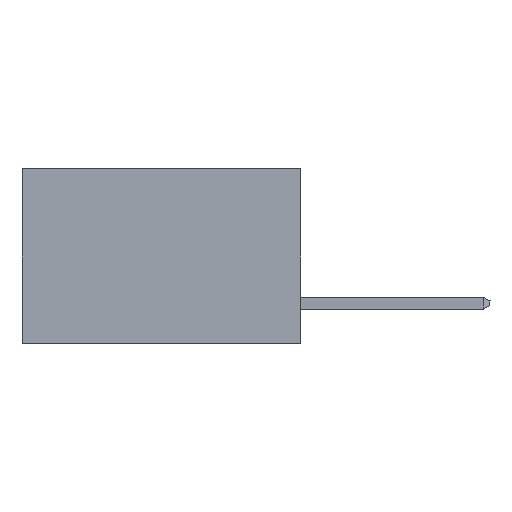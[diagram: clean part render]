
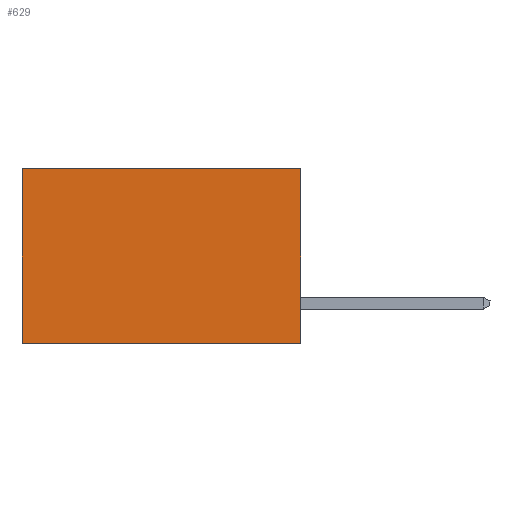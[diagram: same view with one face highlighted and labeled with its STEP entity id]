
A CAD part, left-side view. The second image highlights one B-rep face of the part: STEP entity #629.
In plain terms, the highlighted planar face has unit normal (-1, 0, 0).
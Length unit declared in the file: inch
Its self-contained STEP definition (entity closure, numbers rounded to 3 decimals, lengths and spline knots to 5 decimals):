
#10 = CARTESIAN_POINT ( 'NONE',  ( 0.277, 0., -0.37 ) ) ;
#412 = VECTOR ( 'NONE', #4377, 39.37008 ) ;
#629 = ADVANCED_FACE ( 'NONE', ( #8296 ), #10199, .F. ) ;
#707 = ORIENTED_EDGE ( 'NONE', *, *, #11352, .F. ) ;
#1460 = VECTOR ( 'NONE', #11012, 39.37008 ) ;
#1767 = VECTOR ( 'NONE', #10449, 39.37008 ) ;
#2473 = VERTEX_POINT ( 'NONE', #3828 ) ;
#2776 = AXIS2_PLACEMENT_3D ( 'NONE', #9826, #4956, #4717 ) ;
#3292 = LINE ( 'NONE', #11319, #412 ) ;
#3828 = CARTESIAN_POINT ( 'NONE',  ( 0.277, 0., -0.37 ) ) ;
#4168 = ORIENTED_EDGE ( 'NONE', *, *, #12578, .T. ) ;
#4209 = ORIENTED_EDGE ( 'NONE', *, *, #5076, .F. ) ;
#4377 = DIRECTION ( 'NONE',  ( 0., 0., -1. ) ) ;
#4717 = DIRECTION ( 'NONE',  ( 0., 0., -1. ) ) ;
#4956 = DIRECTION ( 'NONE',  ( 1., 0., 0. ) ) ;
#5076 = EDGE_CURVE ( 'NONE', #2473, #6127, #6480, .T. ) ;
#5223 = LINE ( 'NONE', #5829, #12479 ) ;
#5564 = EDGE_LOOP ( 'NONE', ( #4168, #4209, #707, #8756 ) ) ;
#5798 = DIRECTION ( 'NONE',  ( 0., 1., 0. ) ) ;
#5829 = CARTESIAN_POINT ( 'NONE',  ( 0.277, 0., 0. ) ) ;
#6127 = VERTEX_POINT ( 'NONE', #9019 ) ;
#6455 = EDGE_CURVE ( 'NONE', #10640, #11534, #5223, .T. ) ;
#6480 = LINE ( 'NONE', #10, #1767 ) ;
#7124 = LINE ( 'NONE', #10030, #1460 ) ;
#8296 = FACE_OUTER_BOUND ( 'NONE', #5564, .T. ) ;
#8756 = ORIENTED_EDGE ( 'NONE', *, *, #6455, .T. ) ;
#9019 = CARTESIAN_POINT ( 'NONE',  ( 0.277, 0.59, -0.37 ) ) ;
#9826 = CARTESIAN_POINT ( 'NONE',  ( 0.277, 0., -0.37 ) ) ;
#10030 = CARTESIAN_POINT ( 'NONE',  ( 0.277, 0.59, -0.37 ) ) ;
#10199 = PLANE ( 'NONE',  #2776 ) ;
#10449 = DIRECTION ( 'NONE',  ( 0., 1., 0. ) ) ;
#10476 = CARTESIAN_POINT ( 'NONE',  ( 0.277, 0., 0. ) ) ;
#10545 = CARTESIAN_POINT ( 'NONE',  ( 0.277, 0.59, 0. ) ) ;
#10640 = VERTEX_POINT ( 'NONE', #10476 ) ;
#11012 = DIRECTION ( 'NONE',  ( 0., 0., -1. ) ) ;
#11319 = CARTESIAN_POINT ( 'NONE',  ( 0.277, 0., -0.37 ) ) ;
#11352 = EDGE_CURVE ( 'NONE', #10640, #2473, #3292, .T. ) ;
#11534 = VERTEX_POINT ( 'NONE', #10545 ) ;
#12479 = VECTOR ( 'NONE', #5798, 39.37008 ) ;
#12578 = EDGE_CURVE ( 'NONE', #11534, #6127, #7124, .T. ) ;
